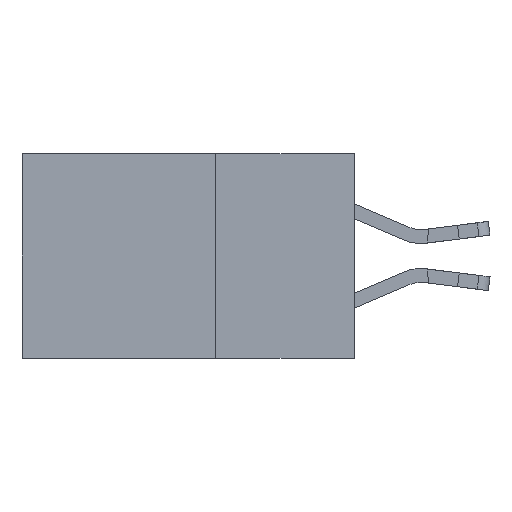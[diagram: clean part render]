
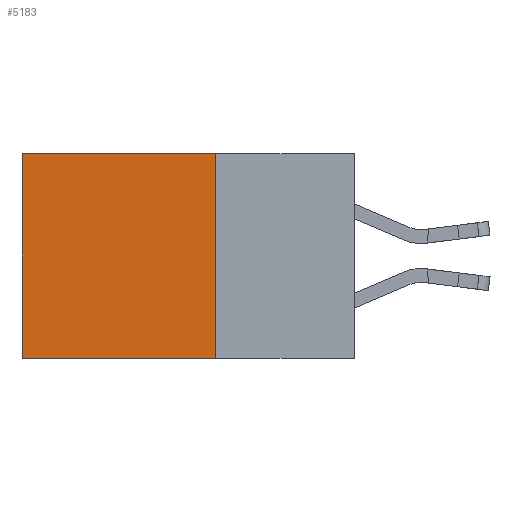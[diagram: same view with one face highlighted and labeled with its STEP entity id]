
A CAD part, left-side view. The second image highlights one B-rep face of the part: STEP entity #5183.
In plain terms, the highlighted planar face has unit normal (-1, 0, 0).
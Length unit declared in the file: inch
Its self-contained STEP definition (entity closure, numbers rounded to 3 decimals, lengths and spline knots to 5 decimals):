
#386 = ORIENTED_EDGE ( 'NONE', *, *, #4181, .F. ) ;
#1693 = CARTESIAN_POINT ( 'NONE',  ( 0.298, 0.25, 0. ) ) ;
#1806 = VECTOR ( 'NONE', #8383, 39.37008 ) ;
#3502 = DIRECTION ( 'NONE',  ( 1., 0., 0. ) ) ;
#3722 = LINE ( 'NONE', #8272, #13847 ) ;
#3820 = VECTOR ( 'NONE', #4025, 39.37008 ) ;
#4025 = DIRECTION ( 'NONE',  ( 0., 0., -1. ) ) ;
#4181 = EDGE_CURVE ( 'NONE', #19074, #9892, #3722, .T. ) ;
#4239 = AXIS2_PLACEMENT_3D ( 'NONE', #1693, #3502, #17904 ) ;
#5049 = PLANE ( 'NONE',  #4239 ) ;
#5183 = ADVANCED_FACE ( 'NONE', ( #18362 ), #5049, .F. ) ;
#5726 = LINE ( 'NONE', #21162, #1806 ) ;
#6555 = VECTOR ( 'NONE', #15079, 39.37008 ) ;
#7392 = LINE ( 'NONE', #7726, #6555 ) ;
#7726 = CARTESIAN_POINT ( 'NONE',  ( 0.298, 0.25, 0. ) ) ;
#8272 = CARTESIAN_POINT ( 'NONE',  ( 0.298, 0.25, -0.37 ) ) ;
#8383 = DIRECTION ( 'NONE',  ( 0., 0., -1. ) ) ;
#9694 = DIRECTION ( 'NONE',  ( 0., 1., 0. ) ) ;
#9892 = VERTEX_POINT ( 'NONE', #16736 ) ;
#11934 = EDGE_LOOP ( 'NONE', ( #12017, #386, #20208, #13062 ) ) ;
#12007 = EDGE_CURVE ( 'NONE', #21128, #9892, #15623, .T. ) ;
#12017 = ORIENTED_EDGE ( 'NONE', *, *, #12007, .T. ) ;
#12699 = EDGE_CURVE ( 'NONE', #13701, #19074, #5726, .T. ) ;
#12965 = CARTESIAN_POINT ( 'NONE',  ( 0.298, 0.6, 0. ) ) ;
#13062 = ORIENTED_EDGE ( 'NONE', *, *, #13529, .T. ) ;
#13529 = EDGE_CURVE ( 'NONE', #13701, #21128, #7392, .T. ) ;
#13701 = VERTEX_POINT ( 'NONE', #20819 ) ;
#13847 = VECTOR ( 'NONE', #9694, 39.37008 ) ;
#15079 = DIRECTION ( 'NONE',  ( 0., 1., 0. ) ) ;
#15623 = LINE ( 'NONE', #12965, #3820 ) ;
#16736 = CARTESIAN_POINT ( 'NONE',  ( 0.298, 0.6, -0.37 ) ) ;
#17904 = DIRECTION ( 'NONE',  ( 0., 0., -1. ) ) ;
#17981 = CARTESIAN_POINT ( 'NONE',  ( 0.298, 0.25, -0.37 ) ) ;
#18362 = FACE_OUTER_BOUND ( 'NONE', #11934, .T. ) ;
#19074 = VERTEX_POINT ( 'NONE', #17981 ) ;
#20208 = ORIENTED_EDGE ( 'NONE', *, *, #12699, .F. ) ;
#20819 = CARTESIAN_POINT ( 'NONE',  ( 0.298, 0.25, 0. ) ) ;
#21128 = VERTEX_POINT ( 'NONE', #22917 ) ;
#21162 = CARTESIAN_POINT ( 'NONE',  ( 0.298, 0.25, 0. ) ) ;
#22917 = CARTESIAN_POINT ( 'NONE',  ( 0.298, 0.6, 0. ) ) ;
